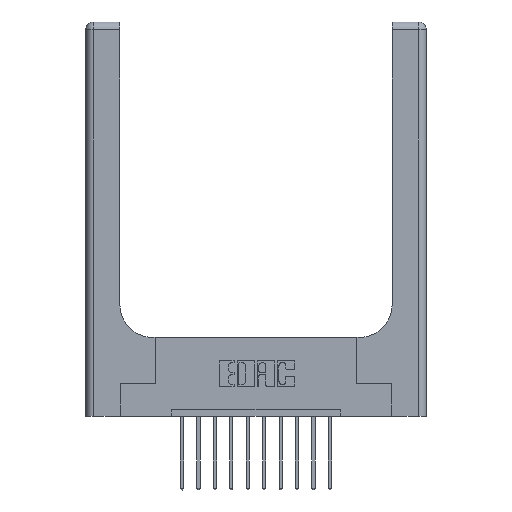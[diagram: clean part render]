
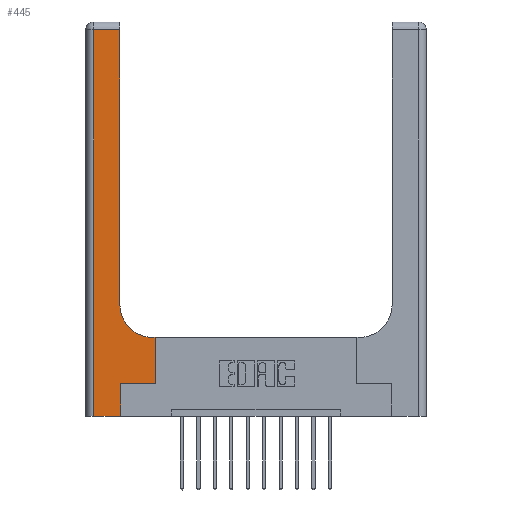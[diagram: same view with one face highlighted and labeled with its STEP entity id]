
A CAD part, top view. The second image highlights one B-rep face of the part: STEP entity #445.
In plain terms, the highlighted planar face has unit normal (0, 0, 1).
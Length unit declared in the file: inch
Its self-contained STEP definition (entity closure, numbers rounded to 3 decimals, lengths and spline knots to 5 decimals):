
#84 = ORIENTED_EDGE ( 'NONE', *, *, #12326, .T. ) ;
#140 = VECTOR ( 'NONE', #792, 39.37008 ) ;
#216 = FACE_OUTER_BOUND ( 'NONE', #9170, .T. ) ;
#445 = ADVANCED_FACE ( 'NONE', ( #216 ), #915, .F. ) ;
#579 = EDGE_CURVE ( 'NONE', #5482, #10995, #13483, .T. ) ;
#675 = VECTOR ( 'NONE', #14842, 39.37008 ) ;
#792 = DIRECTION ( 'NONE',  ( 1., 0., 0. ) ) ;
#915 = PLANE ( 'NONE',  #2458 ) ;
#963 = CARTESIAN_POINT ( 'NONE',  ( 0., 3., 0.37 ) ) ;
#1163 = VECTOR ( 'NONE', #4445, 39.37008 ) ;
#1529 = CARTESIAN_POINT ( 'NONE',  ( 0.528, 0.25, 0.37 ) ) ;
#2053 = AXIS2_PLACEMENT_3D ( 'NONE', #2710, #11170, #3918 ) ;
#2344 = CARTESIAN_POINT ( 'NONE',  ( 0.51, 0.6, 0.37 ) ) ;
#2419 = VECTOR ( 'NONE', #12504, 39.37008 ) ;
#2458 = AXIS2_PLACEMENT_3D ( 'NONE', #963, #7311, #9749 ) ;
#2710 = CARTESIAN_POINT ( 'NONE',  ( 0.51, 0.85, 0.37 ) ) ;
#2994 = ORIENTED_EDGE ( 'NONE', *, *, #7038, .T. ) ;
#3061 = CARTESIAN_POINT ( 'NONE',  ( 0.265, 0., 0.37 ) ) ;
#3082 = DIRECTION ( 'NONE',  ( 0., 1., 0. ) ) ;
#3092 = CARTESIAN_POINT ( 'NONE',  ( 0., 0., 0.37 ) ) ;
#3338 = VERTEX_POINT ( 'NONE', #15123 ) ;
#3414 = VECTOR ( 'NONE', #3082, 39.37008 ) ;
#3577 = EDGE_CURVE ( 'NONE', #15443, #13398, #6395, .T. ) ;
#3918 = DIRECTION ( 'NONE',  ( 1., 0., 0. ) ) ;
#4361 = ORIENTED_EDGE ( 'NONE', *, *, #579, .T. ) ;
#4445 = DIRECTION ( 'NONE',  ( 1., 0., 0. ) ) ;
#4554 = LINE ( 'NONE', #4605, #14239 ) ;
#4605 = CARTESIAN_POINT ( 'NONE',  ( 0.06, 3., 0.37 ) ) ;
#4805 = EDGE_CURVE ( 'NONE', #10216, #9236, #11483, .T. ) ;
#4985 = ORIENTED_EDGE ( 'NONE', *, *, #13592, .T. ) ;
#5482 = VERTEX_POINT ( 'NONE', #13619 ) ;
#5545 = CARTESIAN_POINT ( 'NONE',  ( 0., 2.94, 0.37 ) ) ;
#5555 = VERTEX_POINT ( 'NONE', #13506 ) ;
#5556 = CARTESIAN_POINT ( 'NONE',  ( 0.265, 0., 0.37 ) ) ;
#5648 = ORIENTED_EDGE ( 'NONE', *, *, #4805, .T. ) ;
#5670 = VECTOR ( 'NONE', #6305, 39.37008 ) ;
#6112 = ORIENTED_EDGE ( 'NONE', *, *, #11433, .T. ) ;
#6256 = LINE ( 'NONE', #1529, #5670 ) ;
#6305 = DIRECTION ( 'NONE',  ( 0., 1., 0. ) ) ;
#6354 = CARTESIAN_POINT ( 'NONE',  ( 0.26, 0.6, 0.37 ) ) ;
#6395 = LINE ( 'NONE', #6354, #2419 ) ;
#6638 = LINE ( 'NONE', #5556, #3414 ) ;
#7038 = EDGE_CURVE ( 'NONE', #3338, #9463, #10397, .T. ) ;
#7311 = DIRECTION ( 'NONE',  ( 0., 0., -1. ) ) ;
#8820 = ORIENTED_EDGE ( 'NONE', *, *, #15211, .T. ) ;
#8943 = ORIENTED_EDGE ( 'NONE', *, *, #15063, .T. ) ;
#9170 = EDGE_LOOP ( 'NONE', ( #5648, #6112, #84, #2994, #8820, #4361, #8943, #12875, #4985 ) ) ;
#9183 = DIRECTION ( 'NONE',  ( -1., 0., 0. ) ) ;
#9236 = VERTEX_POINT ( 'NONE', #14696 ) ;
#9463 = VERTEX_POINT ( 'NONE', #3061 ) ;
#9467 = DIRECTION ( 'NONE',  ( 0., -1., 0. ) ) ;
#9749 = DIRECTION ( 'NONE',  ( -1., 0., 0. ) ) ;
#9962 = CARTESIAN_POINT ( 'NONE',  ( 0.26, 3., 0.37 ) ) ;
#10216 = VERTEX_POINT ( 'NONE', #12017 ) ;
#10397 = LINE ( 'NONE', #3092, #140 ) ;
#10995 = VERTEX_POINT ( 'NONE', #15465 ) ;
#11170 = DIRECTION ( 'NONE',  ( 0., 0., -1. ) ) ;
#11433 = EDGE_CURVE ( 'NONE', #9236, #5555, #15026, .T. ) ;
#11483 = LINE ( 'NONE', #9962, #675 ) ;
#11717 = CARTESIAN_POINT ( 'NONE',  ( 0.265, 0.25, 0.37 ) ) ;
#12017 = CARTESIAN_POINT ( 'NONE',  ( 0.26, 0.85, 0.37 ) ) ;
#12117 = CARTESIAN_POINT ( 'NONE',  ( 0.528, 0.6, 0.37 ) ) ;
#12326 = EDGE_CURVE ( 'NONE', #5555, #3338, #4554, .T. ) ;
#12504 = DIRECTION ( 'NONE',  ( -1., 0., 0. ) ) ;
#12875 = ORIENTED_EDGE ( 'NONE', *, *, #3577, .T. ) ;
#13398 = VERTEX_POINT ( 'NONE', #2344 ) ;
#13483 = LINE ( 'NONE', #11717, #1163 ) ;
#13498 = CIRCLE ( 'NONE', #2053, 0.25 ) ;
#13506 = CARTESIAN_POINT ( 'NONE',  ( 0.06, 2.94, 0.37 ) ) ;
#13592 = EDGE_CURVE ( 'NONE', #13398, #10216, #13498, .T. ) ;
#13619 = CARTESIAN_POINT ( 'NONE',  ( 0.265, 0.25, 0.37 ) ) ;
#14239 = VECTOR ( 'NONE', #9467, 39.37008 ) ;
#14696 = CARTESIAN_POINT ( 'NONE',  ( 0.26, 2.94, 0.37 ) ) ;
#14842 = DIRECTION ( 'NONE',  ( 0., 1., 0. ) ) ;
#15026 = LINE ( 'NONE', #5545, #15222 ) ;
#15063 = EDGE_CURVE ( 'NONE', #10995, #15443, #6256, .T. ) ;
#15123 = CARTESIAN_POINT ( 'NONE',  ( 0.06, 0., 0.37 ) ) ;
#15211 = EDGE_CURVE ( 'NONE', #9463, #5482, #6638, .T. ) ;
#15222 = VECTOR ( 'NONE', #9183, 39.37008 ) ;
#15443 = VERTEX_POINT ( 'NONE', #12117 ) ;
#15465 = CARTESIAN_POINT ( 'NONE',  ( 0.528, 0.25, 0.37 ) ) ;
